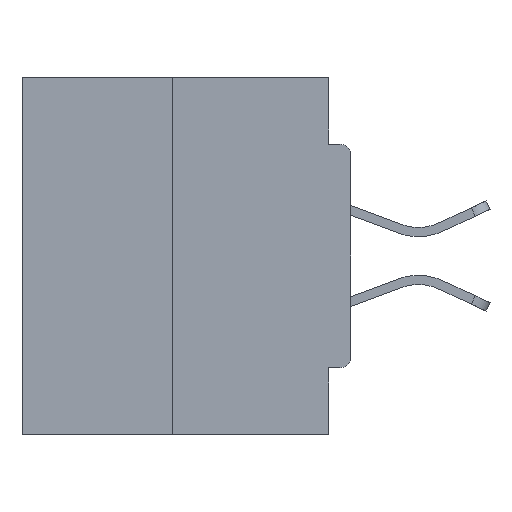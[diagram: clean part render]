
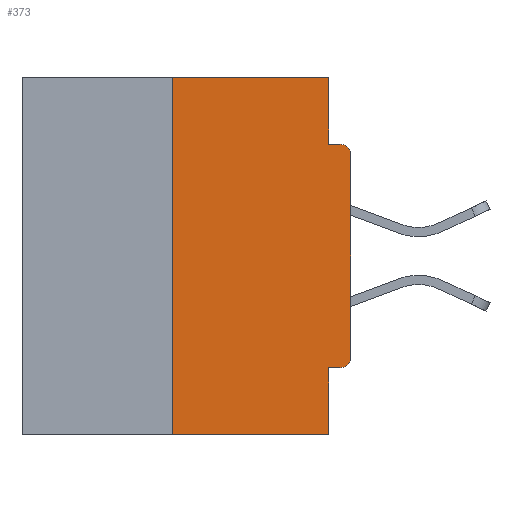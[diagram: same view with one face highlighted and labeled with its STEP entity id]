
A CAD part, left-side view. The second image highlights one B-rep face of the part: STEP entity #373.
In plain terms, the highlighted planar face has unit normal (-1, 0, 0).
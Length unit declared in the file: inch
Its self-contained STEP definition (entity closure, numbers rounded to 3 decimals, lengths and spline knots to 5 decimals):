
#152 = CARTESIAN_POINT ( 'NONE',  ( 0., 0.46, -0.5 ) ) ;
#313 = ORIENTED_EDGE ( 'NONE', *, *, #11849, .F. ) ;
#367 = CARTESIAN_POINT ( 'NONE',  ( 0., 0.25, 0. ) ) ;
#373 = ADVANCED_FACE ( 'NONE', ( #14360 ), #6698, .F. ) ;
#1127 = DIRECTION ( 'NONE',  ( 0., 0., 1. ) ) ;
#1293 = CARTESIAN_POINT ( 'NONE',  ( 0., 0.015, -0.0935 ) ) ;
#1895 = CARTESIAN_POINT ( 'NONE',  ( 0., 0., 0. ) ) ;
#2262 = LINE ( 'NONE', #1895, #4330 ) ;
#2476 = CARTESIAN_POINT ( 'NONE',  ( 0., 0.25, -0.5 ) ) ;
#2530 = CARTESIAN_POINT ( 'NONE',  ( 0., 0., -0.3915 ) ) ;
#2776 = VERTEX_POINT ( 'NONE', #367 ) ;
#3217 = AXIS2_PLACEMENT_3D ( 'NONE', #25077, #11813, #4013 ) ;
#3402 = ORIENTED_EDGE ( 'NONE', *, *, #34138, .F. ) ;
#4013 = DIRECTION ( 'NONE',  ( 0., 0., -1. ) ) ;
#4036 = VERTEX_POINT ( 'NONE', #2476 ) ;
#4330 = VECTOR ( 'NONE', #31038, 39.37008 ) ;
#4336 = DIRECTION ( 'NONE',  ( 0., 1., 0. ) ) ;
#4570 = VECTOR ( 'NONE', #1127, 39.37008 ) ;
#4606 = EDGE_CURVE ( 'NONE', #22441, #7335, #2262, .T. ) ;
#4742 = ORIENTED_EDGE ( 'NONE', *, *, #23470, .T. ) ;
#5439 = DIRECTION ( 'NONE',  ( 0., -1., 0. ) ) ;
#5834 = CARTESIAN_POINT ( 'NONE',  ( 0., 0.25, 0. ) ) ;
#6073 = LINE ( 'NONE', #32672, #11388 ) ;
#6698 = PLANE ( 'NONE',  #11543 ) ;
#6858 = CARTESIAN_POINT ( 'NONE',  ( 0., 0., -0.4065 ) ) ;
#7262 = CARTESIAN_POINT ( 'NONE',  ( 0., 0.031, -0.4065 ) ) ;
#7335 = VERTEX_POINT ( 'NONE', #24054 ) ;
#7682 = EDGE_CURVE ( 'NONE', #4036, #2776, #9468, .T. ) ;
#8066 = CARTESIAN_POINT ( 'NONE',  ( 0., 0.031, -0.5 ) ) ;
#8236 = VECTOR ( 'NONE', #25304, 39.37008 ) ;
#9221 = CARTESIAN_POINT ( 'NONE',  ( 0., 0.46, 0. ) ) ;
#9468 = LINE ( 'NONE', #5834, #4570 ) ;
#9683 = EDGE_CURVE ( 'NONE', #15913, #11635, #26268, .T. ) ;
#11318 = ORIENTED_EDGE ( 'NONE', *, *, #30573, .F. ) ;
#11388 = VECTOR ( 'NONE', #32785, 39.37008 ) ;
#11463 = LINE ( 'NONE', #33905, #13977 ) ;
#11543 = AXIS2_PLACEMENT_3D ( 'NONE', #9221, #25127, #11980 ) ;
#11635 = VERTEX_POINT ( 'NONE', #1293 ) ;
#11813 = DIRECTION ( 'NONE',  ( -1., 0., 0. ) ) ;
#11849 = EDGE_CURVE ( 'NONE', #30831, #12468, #11463, .T. ) ;
#11980 = DIRECTION ( 'NONE',  ( 0., 0., -1. ) ) ;
#12031 = VECTOR ( 'NONE', #4336, 39.37008 ) ;
#12389 = CARTESIAN_POINT ( 'NONE',  ( 0., 0.031, 0. ) ) ;
#12468 = VERTEX_POINT ( 'NONE', #8066 ) ;
#13977 = VECTOR ( 'NONE', #23458, 39.37008 ) ;
#14330 = LINE ( 'NONE', #152, #28747 ) ;
#14360 = FACE_OUTER_BOUND ( 'NONE', #21146, .T. ) ;
#14585 = ORIENTED_EDGE ( 'NONE', *, *, #32912, .F. ) ;
#14730 = DIRECTION ( 'NONE',  ( 0., 0., -1. ) ) ;
#14756 = DIRECTION ( 'NONE',  ( 0., -1., 0. ) ) ;
#15242 = LINE ( 'NONE', #17237, #8236 ) ;
#15906 = CARTESIAN_POINT ( 'NONE',  ( 0., 0.031, -0.0935 ) ) ;
#15913 = VERTEX_POINT ( 'NONE', #15906 ) ;
#16761 = EDGE_CURVE ( 'NONE', #7335, #11635, #29345, .T. ) ;
#17237 = CARTESIAN_POINT ( 'NONE',  ( 0., 0.46, 0. ) ) ;
#18507 = ORIENTED_EDGE ( 'NONE', *, *, #4606, .T. ) ;
#18623 = AXIS2_PLACEMENT_3D ( 'NONE', #24877, #30327, #14730 ) ;
#19069 = LINE ( 'NONE', #6858, #12031 ) ;
#19257 = VECTOR ( 'NONE', #14756, 39.37008 ) ;
#20464 = ORIENTED_EDGE ( 'NONE', *, *, #16761, .T. ) ;
#21146 = EDGE_LOOP ( 'NONE', ( #3402, #29578, #28423, #313, #14585, #4742, #18507, #20464, #22928, #11318 ) ) ;
#22441 = VERTEX_POINT ( 'NONE', #2530 ) ;
#22928 = ORIENTED_EDGE ( 'NONE', *, *, #9683, .F. ) ;
#23458 = DIRECTION ( 'NONE',  ( 0., 0., -1. ) ) ;
#23470 = EDGE_CURVE ( 'NONE', #24332, #22441, #25970, .T. ) ;
#24054 = CARTESIAN_POINT ( 'NONE',  ( 0., 0., -0.1085 ) ) ;
#24332 = VERTEX_POINT ( 'NONE', #26443 ) ;
#24629 = EDGE_CURVE ( 'NONE', #4036, #12468, #14330, .T. ) ;
#24877 = CARTESIAN_POINT ( 'NONE',  ( 0., 0.015, -0.3915 ) ) ;
#24902 = CARTESIAN_POINT ( 'NONE',  ( 0., 0., -0.0935 ) ) ;
#25077 = CARTESIAN_POINT ( 'NONE',  ( 0., 0.015, -0.1085 ) ) ;
#25127 = DIRECTION ( 'NONE',  ( 1., 0., 0. ) ) ;
#25304 = DIRECTION ( 'NONE',  ( 0., -1., 0. ) ) ;
#25970 = CIRCLE ( 'NONE', #18623, 0.015 ) ;
#26268 = LINE ( 'NONE', #24902, #19257 ) ;
#26443 = CARTESIAN_POINT ( 'NONE',  ( 0., 0.015, -0.4065 ) ) ;
#28423 = ORIENTED_EDGE ( 'NONE', *, *, #24629, .T. ) ;
#28747 = VECTOR ( 'NONE', #5439, 39.37008 ) ;
#29345 = CIRCLE ( 'NONE', #3217, 0.015 ) ;
#29578 = ORIENTED_EDGE ( 'NONE', *, *, #7682, .F. ) ;
#30327 = DIRECTION ( 'NONE',  ( -1., 0., 0. ) ) ;
#30573 = EDGE_CURVE ( 'NONE', #31383, #15913, #6073, .T. ) ;
#30831 = VERTEX_POINT ( 'NONE', #7262 ) ;
#31038 = DIRECTION ( 'NONE',  ( 0., 0., 1. ) ) ;
#31383 = VERTEX_POINT ( 'NONE', #12389 ) ;
#32672 = CARTESIAN_POINT ( 'NONE',  ( 0., 0.031, 0. ) ) ;
#32785 = DIRECTION ( 'NONE',  ( 0., 0., -1. ) ) ;
#32912 = EDGE_CURVE ( 'NONE', #24332, #30831, #19069, .T. ) ;
#33905 = CARTESIAN_POINT ( 'NONE',  ( 0., 0.031, -0.5 ) ) ;
#34138 = EDGE_CURVE ( 'NONE', #2776, #31383, #15242, .T. ) ;
